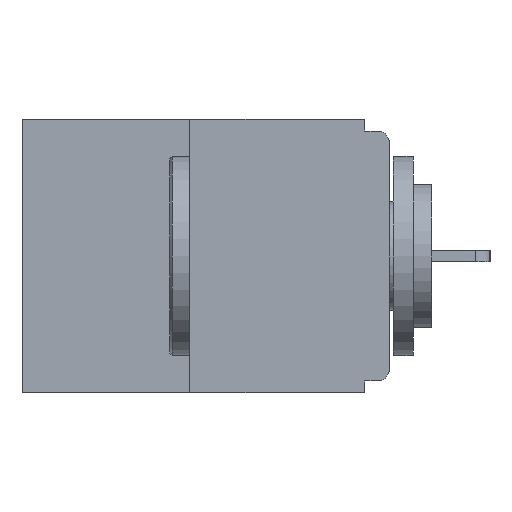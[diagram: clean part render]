
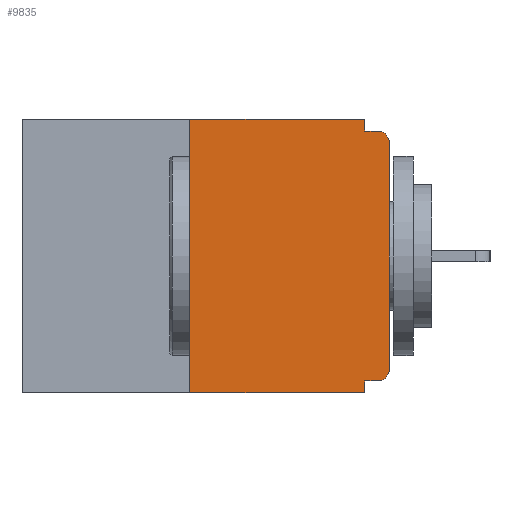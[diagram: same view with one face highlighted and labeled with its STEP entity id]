
A CAD part, left-side view. The second image highlights one B-rep face of the part: STEP entity #9835.
In plain terms, the highlighted planar face has unit normal (-1, 0, 0).
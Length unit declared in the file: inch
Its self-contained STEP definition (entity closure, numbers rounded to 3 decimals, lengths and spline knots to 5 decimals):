
#90 = CARTESIAN_POINT ( 'NONE',  ( 0., 0.25, 0. ) ) ;
#234 = VERTEX_POINT ( 'NONE', #15583 ) ;
#278 = EDGE_CURVE ( 'NONE', #15742, #6533, #5813, .T. ) ;
#427 = DIRECTION ( 'NONE',  ( 0., -1., 0. ) ) ;
#1565 = VECTOR ( 'NONE', #20112, 39.37008 ) ;
#1812 = CARTESIAN_POINT ( 'NONE',  ( 0., 0.46, -0.343 ) ) ;
#1856 = CIRCLE ( 'NONE', #14136, 0.015 ) ;
#2053 = EDGE_CURVE ( 'NONE', #9958, #17874, #3021, .T. ) ;
#2625 = CARTESIAN_POINT ( 'NONE',  ( 0., 0., -0.03 ) ) ;
#2964 = DIRECTION ( 'NONE',  ( -1., 0., 0. ) ) ;
#2995 = EDGE_CURVE ( 'NONE', #5395, #234, #19439, .T. ) ;
#3021 = LINE ( 'NONE', #3631, #11388 ) ;
#3128 = VECTOR ( 'NONE', #14534, 39.37008 ) ;
#3156 = VECTOR ( 'NONE', #6777, 39.37008 ) ;
#3197 = CARTESIAN_POINT ( 'NONE',  ( 0., 0.015, -0.313 ) ) ;
#3613 = CARTESIAN_POINT ( 'NONE',  ( 0., 0., -0.015 ) ) ;
#3631 = CARTESIAN_POINT ( 'NONE',  ( 0., 0.031, 0. ) ) ;
#3714 = CARTESIAN_POINT ( 'NONE',  ( 0., 0.46, 0. ) ) ;
#3725 = EDGE_CURVE ( 'NONE', #4102, #9958, #17440, .T. ) ;
#4102 = VERTEX_POINT ( 'NONE', #90 ) ;
#4801 = DIRECTION ( 'NONE',  ( 0., 0., -1. ) ) ;
#5092 = VECTOR ( 'NONE', #427, 39.37008 ) ;
#5175 = VERTEX_POINT ( 'NONE', #16960 ) ;
#5379 = DIRECTION ( 'NONE',  ( 1., 0., 0. ) ) ;
#5395 = VERTEX_POINT ( 'NONE', #17814 ) ;
#5511 = ORIENTED_EDGE ( 'NONE', *, *, #17728, .T. ) ;
#5813 = LINE ( 'NONE', #1812, #1565 ) ;
#5885 = CARTESIAN_POINT ( 'NONE',  ( 0., 0.25, -0.343 ) ) ;
#6230 = ORIENTED_EDGE ( 'NONE', *, *, #278, .T. ) ;
#6533 = VERTEX_POINT ( 'NONE', #18807 ) ;
#6699 = CIRCLE ( 'NONE', #13435, 0.015 ) ;
#6777 = DIRECTION ( 'NONE',  ( 0., 0., 1. ) ) ;
#7369 = LINE ( 'NONE', #11430, #3156 ) ;
#7810 = VECTOR ( 'NONE', #12030, 39.37008 ) ;
#7939 = ORIENTED_EDGE ( 'NONE', *, *, #3725, .F. ) ;
#8440 = ORIENTED_EDGE ( 'NONE', *, *, #18901, .F. ) ;
#8502 = VECTOR ( 'NONE', #15508, 39.37008 ) ;
#8964 = DIRECTION ( 'NONE',  ( 0., 0., -1. ) ) ;
#9066 = DIRECTION ( 'NONE',  ( 0., 1., 0. ) ) ;
#9434 = VERTEX_POINT ( 'NONE', #16841 ) ;
#9835 = ADVANCED_FACE ( 'NONE', ( #12882 ), #13157, .F. ) ;
#9877 = CARTESIAN_POINT ( 'NONE',  ( 0., 0.031, -0.015 ) ) ;
#9958 = VERTEX_POINT ( 'NONE', #19512 ) ;
#10320 = CARTESIAN_POINT ( 'NONE',  ( 0., 0., -0.328 ) ) ;
#10446 = ORIENTED_EDGE ( 'NONE', *, *, #17886, .F. ) ;
#10478 = CARTESIAN_POINT ( 'NONE',  ( 0., 0.031, -0.343 ) ) ;
#10919 = ORIENTED_EDGE ( 'NONE', *, *, #2053, .F. ) ;
#11108 = VERTEX_POINT ( 'NONE', #2625 ) ;
#11388 = VECTOR ( 'NONE', #8964, 39.37008 ) ;
#11430 = CARTESIAN_POINT ( 'NONE',  ( 0., 0., 0. ) ) ;
#11974 = LINE ( 'NONE', #3613, #3128 ) ;
#12030 = DIRECTION ( 'NONE',  ( 0., 0., -1. ) ) ;
#12106 = EDGE_CURVE ( 'NONE', #11108, #9434, #6699, .T. ) ;
#12356 = CARTESIAN_POINT ( 'NONE',  ( 0., 0.015, -0.03 ) ) ;
#12596 = ORIENTED_EDGE ( 'NONE', *, *, #12106, .T. ) ;
#12638 = LINE ( 'NONE', #15440, #8502 ) ;
#12882 = FACE_OUTER_BOUND ( 'NONE', #19975, .T. ) ;
#13157 = PLANE ( 'NONE',  #18217 ) ;
#13329 = ORIENTED_EDGE ( 'NONE', *, *, #2995, .F. ) ;
#13435 = AXIS2_PLACEMENT_3D ( 'NONE', #12356, #2964, #13903 ) ;
#13622 = EDGE_CURVE ( 'NONE', #5175, #11108, #7369, .T. ) ;
#13903 = DIRECTION ( 'NONE',  ( 0., 0., -1. ) ) ;
#14131 = DIRECTION ( 'NONE',  ( -1., 0., 0. ) ) ;
#14136 = AXIS2_PLACEMENT_3D ( 'NONE', #3197, #14131, #4801 ) ;
#14520 = EDGE_CURVE ( 'NONE', #234, #6533, #16047, .T. ) ;
#14534 = DIRECTION ( 'NONE',  ( 0., -1., 0. ) ) ;
#15009 = ORIENTED_EDGE ( 'NONE', *, *, #14520, .F. ) ;
#15417 = CARTESIAN_POINT ( 'NONE',  ( 0., 0.46, 0. ) ) ;
#15440 = CARTESIAN_POINT ( 'NONE',  ( 0., 0.25, 0. ) ) ;
#15442 = VECTOR ( 'NONE', #9066, 39.37008 ) ;
#15508 = DIRECTION ( 'NONE',  ( 0., 0., 1. ) ) ;
#15583 = CARTESIAN_POINT ( 'NONE',  ( 0., 0.031, -0.328 ) ) ;
#15719 = ORIENTED_EDGE ( 'NONE', *, *, #13622, .T. ) ;
#15742 = VERTEX_POINT ( 'NONE', #5885 ) ;
#16047 = LINE ( 'NONE', #10478, #7810 ) ;
#16247 = DIRECTION ( 'NONE',  ( 0., 0., -1. ) ) ;
#16841 = CARTESIAN_POINT ( 'NONE',  ( 0., 0.015, -0.015 ) ) ;
#16960 = CARTESIAN_POINT ( 'NONE',  ( 0., 0., -0.313 ) ) ;
#17440 = LINE ( 'NONE', #15417, #5092 ) ;
#17728 = EDGE_CURVE ( 'NONE', #5395, #5175, #1856, .T. ) ;
#17814 = CARTESIAN_POINT ( 'NONE',  ( 0., 0.015, -0.328 ) ) ;
#17874 = VERTEX_POINT ( 'NONE', #9877 ) ;
#17886 = EDGE_CURVE ( 'NONE', #17874, #9434, #11974, .T. ) ;
#18217 = AXIS2_PLACEMENT_3D ( 'NONE', #3714, #5379, #16247 ) ;
#18807 = CARTESIAN_POINT ( 'NONE',  ( 0., 0.031, -0.343 ) ) ;
#18901 = EDGE_CURVE ( 'NONE', #15742, #4102, #12638, .T. ) ;
#19439 = LINE ( 'NONE', #10320, #15442 ) ;
#19512 = CARTESIAN_POINT ( 'NONE',  ( 0., 0.031, 0. ) ) ;
#19975 = EDGE_LOOP ( 'NONE', ( #7939, #8440, #6230, #15009, #13329, #5511, #15719, #12596, #10446, #10919 ) ) ;
#20112 = DIRECTION ( 'NONE',  ( 0., -1., 0. ) ) ;
